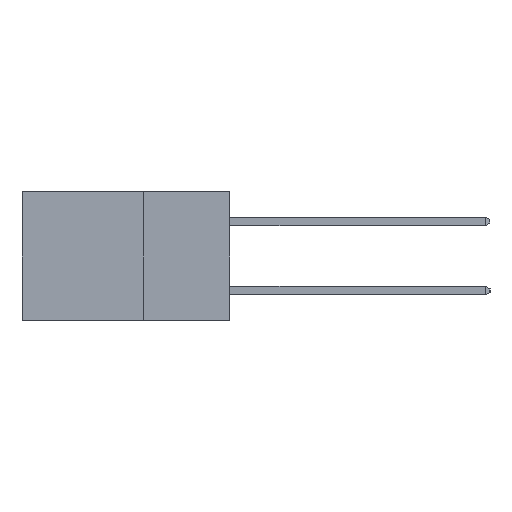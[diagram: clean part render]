
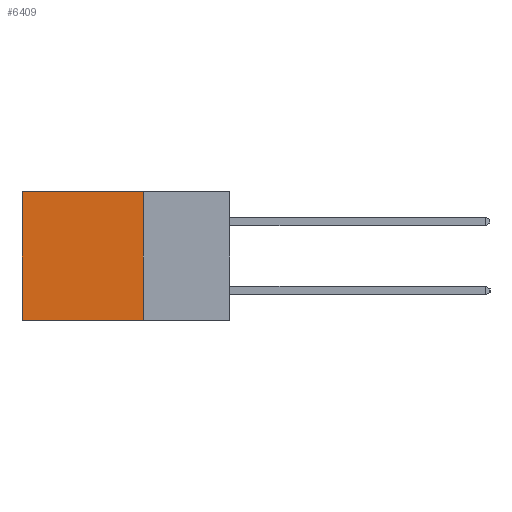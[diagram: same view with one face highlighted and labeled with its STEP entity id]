
A CAD part, left-side view. The second image highlights one B-rep face of the part: STEP entity #6409.
In plain terms, the highlighted planar face has unit normal (-1, 0, 0).
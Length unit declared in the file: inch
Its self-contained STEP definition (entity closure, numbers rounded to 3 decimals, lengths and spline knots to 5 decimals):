
#53 = CARTESIAN_POINT ( 'NONE',  ( 0.2615, 0.25, -0.37 ) ) ;
#83 = CARTESIAN_POINT ( 'NONE',  ( 0.2615, 0.25, -0.37 ) ) ;
#224 = ORIENTED_EDGE ( 'NONE', *, *, #5250, .F. ) ;
#313 = CARTESIAN_POINT ( 'NONE',  ( 0.2615, 0.25, -0.37 ) ) ;
#334 = CARTESIAN_POINT ( 'NONE',  ( 0.2615, 0.6, -0.37 ) ) ;
#580 = CARTESIAN_POINT ( 'NONE',  ( 0.2615, 0.6, -0.37 ) ) ;
#1014 = VERTEX_POINT ( 'NONE', #3431 ) ;
#1821 = LINE ( 'NONE', #580, #10296 ) ;
#1867 = LINE ( 'NONE', #83, #8098 ) ;
#2012 = LINE ( 'NONE', #6984, #7731 ) ;
#2567 = PLANE ( 'NONE',  #3654 ) ;
#2607 = DIRECTION ( 'NONE',  ( 0., 0., -1. ) ) ;
#2682 = CARTESIAN_POINT ( 'NONE',  ( 0.2615, 0.25, 0. ) ) ;
#2774 = EDGE_LOOP ( 'NONE', ( #8957, #7640, #224, #10256 ) ) ;
#3431 = CARTESIAN_POINT ( 'NONE',  ( 0.2615, 0.25, -0.37 ) ) ;
#3654 = AXIS2_PLACEMENT_3D ( 'NONE', #53, #7477, #2607 ) ;
#3762 = DIRECTION ( 'NONE',  ( 0., 1., 0. ) ) ;
#4126 = CARTESIAN_POINT ( 'NONE',  ( 0.2615, 0.6, 0. ) ) ;
#4637 = FACE_OUTER_BOUND ( 'NONE', #2774, .T. ) ;
#5030 = VECTOR ( 'NONE', #5284, 39.37008 ) ;
#5250 = EDGE_CURVE ( 'NONE', #6974, #1014, #5542, .T. ) ;
#5284 = DIRECTION ( 'NONE',  ( 0., 0., -1. ) ) ;
#5542 = LINE ( 'NONE', #313, #5030 ) ;
#5951 = VERTEX_POINT ( 'NONE', #334 ) ;
#6296 = VERTEX_POINT ( 'NONE', #4126 ) ;
#6409 = ADVANCED_FACE ( 'NONE', ( #4637 ), #2567, .F. ) ;
#6735 = DIRECTION ( 'NONE',  ( 0., 1., 0. ) ) ;
#6920 = EDGE_CURVE ( 'NONE', #1014, #5951, #1867, .T. ) ;
#6974 = VERTEX_POINT ( 'NONE', #2682 ) ;
#6984 = CARTESIAN_POINT ( 'NONE',  ( 0.2615, 0.25, 0. ) ) ;
#7162 = EDGE_CURVE ( 'NONE', #6974, #6296, #2012, .T. ) ;
#7477 = DIRECTION ( 'NONE',  ( 1., 0., 0. ) ) ;
#7640 = ORIENTED_EDGE ( 'NONE', *, *, #6920, .F. ) ;
#7731 = VECTOR ( 'NONE', #3762, 39.37008 ) ;
#8098 = VECTOR ( 'NONE', #6735, 39.37008 ) ;
#8957 = ORIENTED_EDGE ( 'NONE', *, *, #10145, .T. ) ;
#9456 = DIRECTION ( 'NONE',  ( 0., 0., -1. ) ) ;
#10145 = EDGE_CURVE ( 'NONE', #6296, #5951, #1821, .T. ) ;
#10256 = ORIENTED_EDGE ( 'NONE', *, *, #7162, .T. ) ;
#10296 = VECTOR ( 'NONE', #9456, 39.37008 ) ;
